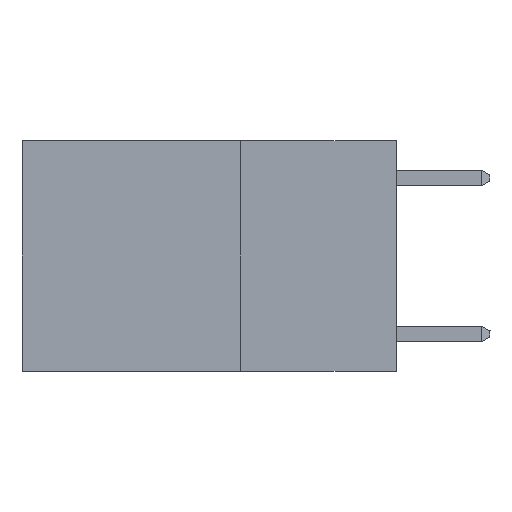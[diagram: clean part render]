
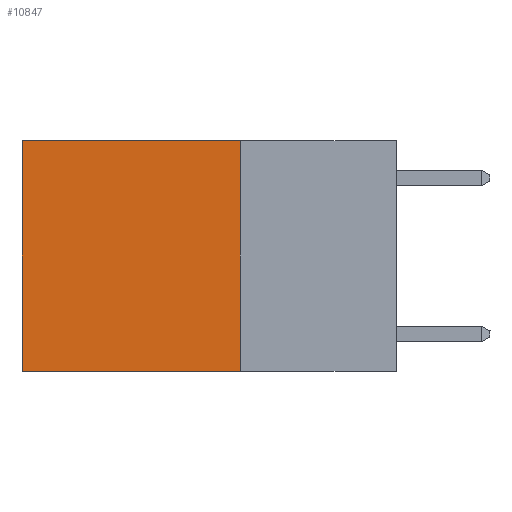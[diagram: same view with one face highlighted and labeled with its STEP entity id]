
A CAD part, left-side view. The second image highlights one B-rep face of the part: STEP entity #10847.
In plain terms, the highlighted planar face has unit normal (-1, 0, 0).
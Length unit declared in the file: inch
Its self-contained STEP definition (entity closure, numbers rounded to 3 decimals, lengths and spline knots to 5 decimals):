
#569 = ORIENTED_EDGE ( 'NONE', *, *, #3668, .T. ) ;
#996 = CARTESIAN_POINT ( 'NONE',  ( 0.2625, 0.25, -0.37 ) ) ;
#1095 = CARTESIAN_POINT ( 'NONE',  ( 0.2625, 0.25, 0. ) ) ;
#2712 = EDGE_LOOP ( 'NONE', ( #569, #8377, #6326, #7747 ) ) ;
#3597 = VECTOR ( 'NONE', #7921, 39.37008 ) ;
#3668 = EDGE_CURVE ( 'NONE', #12052, #10881, #8965, .T. ) ;
#3968 = CARTESIAN_POINT ( 'NONE',  ( 0.2625, 0.6, -0.37 ) ) ;
#4138 = AXIS2_PLACEMENT_3D ( 'NONE', #5826, #11559, #5875 ) ;
#4192 = DIRECTION ( 'NONE',  ( 0., 1., 0. ) ) ;
#4468 = CARTESIAN_POINT ( 'NONE',  ( 0.2625, 0.6, 0. ) ) ;
#4906 = PLANE ( 'NONE',  #4138 ) ;
#5021 = VECTOR ( 'NONE', #7273, 39.37008 ) ;
#5024 = CARTESIAN_POINT ( 'NONE',  ( 0.2625, 0.25, -0.37 ) ) ;
#5135 = CARTESIAN_POINT ( 'NONE',  ( 0.2625, 0.25, 0. ) ) ;
#5286 = LINE ( 'NONE', #5135, #9765 ) ;
#5514 = EDGE_CURVE ( 'NONE', #6568, #9666, #12576, .T. ) ;
#5826 = CARTESIAN_POINT ( 'NONE',  ( 0.2625, 0.25, 0. ) ) ;
#5875 = DIRECTION ( 'NONE',  ( 0., 0., -1. ) ) ;
#6127 = CARTESIAN_POINT ( 'NONE',  ( 0.2625, 0.6, 0. ) ) ;
#6326 = ORIENTED_EDGE ( 'NONE', *, *, #5514, .F. ) ;
#6530 = EDGE_CURVE ( 'NONE', #9666, #10881, #10938, .T. ) ;
#6568 = VERTEX_POINT ( 'NONE', #1095 ) ;
#6603 = EDGE_CURVE ( 'NONE', #6568, #12052, #5286, .T. ) ;
#7273 = DIRECTION ( 'NONE',  ( 0., 0., -1. ) ) ;
#7747 = ORIENTED_EDGE ( 'NONE', *, *, #6603, .T. ) ;
#7921 = DIRECTION ( 'NONE',  ( 0., 1., 0. ) ) ;
#8370 = FACE_OUTER_BOUND ( 'NONE', #2712, .T. ) ;
#8377 = ORIENTED_EDGE ( 'NONE', *, *, #6530, .F. ) ;
#8965 = LINE ( 'NONE', #4468, #11170 ) ;
#9666 = VERTEX_POINT ( 'NONE', #5024 ) ;
#9765 = VECTOR ( 'NONE', #4192, 39.37008 ) ;
#10847 = ADVANCED_FACE ( 'NONE', ( #8370 ), #4906, .F. ) ;
#10881 = VERTEX_POINT ( 'NONE', #3968 ) ;
#10938 = LINE ( 'NONE', #996, #3597 ) ;
#11170 = VECTOR ( 'NONE', #12057, 39.37008 ) ;
#11559 = DIRECTION ( 'NONE',  ( 1., 0., 0. ) ) ;
#11963 = CARTESIAN_POINT ( 'NONE',  ( 0.2625, 0.25, 0. ) ) ;
#12052 = VERTEX_POINT ( 'NONE', #6127 ) ;
#12057 = DIRECTION ( 'NONE',  ( 0., 0., -1. ) ) ;
#12576 = LINE ( 'NONE', #11963, #5021 ) ;
